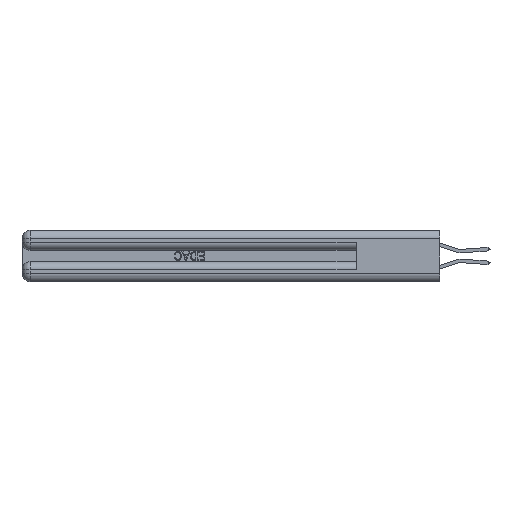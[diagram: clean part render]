
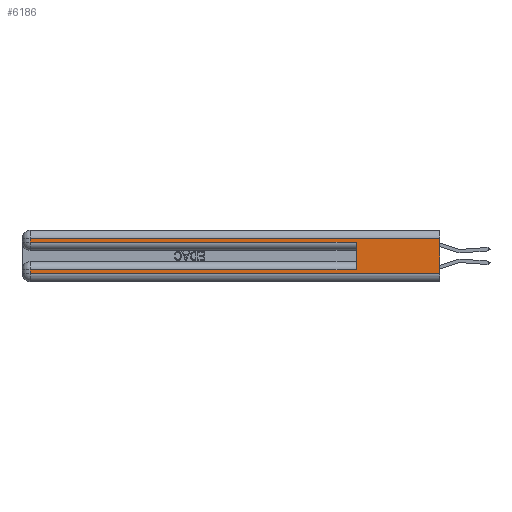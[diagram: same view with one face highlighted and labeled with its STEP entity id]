
A CAD part, left-side view. The second image highlights one B-rep face of the part: STEP entity #6186.
In plain terms, the highlighted planar face has unit normal (-1, 0, 0).
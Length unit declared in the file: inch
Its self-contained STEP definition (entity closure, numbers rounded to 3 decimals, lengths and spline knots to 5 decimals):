
#1685 = VERTEX_POINT ( 'NONE', #13729 ) ;
#1734 = ORIENTED_EDGE ( 'NONE', *, *, #13309, .T. ) ;
#2206 = DIRECTION ( 'NONE',  ( 0., 1., 0. ) ) ;
#2446 = DIRECTION ( 'NONE',  ( 1., 0., 0. ) ) ;
#2831 = EDGE_CURVE ( 'NONE', #9744, #1685, #5831, .T. ) ;
#3284 = VECTOR ( 'NONE', #41558, 39.37008 ) ;
#4957 = CARTESIAN_POINT ( 'NONE',  ( 0., 0.6, 0.085 ) ) ;
#5831 = LINE ( 'NONE', #7526, #36513 ) ;
#6186 = ADVANCED_FACE ( 'NONE', ( #16926 ), #17449, .F. ) ;
#6455 = VECTOR ( 'NONE', #2206, 39.37008 ) ;
#7526 = CARTESIAN_POINT ( 'NONE',  ( 0., 0., 0.285 ) ) ;
#8013 = LINE ( 'NONE', #31637, #43025 ) ;
#9462 = EDGE_CURVE ( 'NONE', #42711, #1685, #14419, .T. ) ;
#9478 = DIRECTION ( 'NONE',  ( 0., 0., -1. ) ) ;
#9744 = VERTEX_POINT ( 'NONE', #45219 ) ;
#9924 = DIRECTION ( 'NONE',  ( 0., 0., -1. ) ) ;
#10524 = ORIENTED_EDGE ( 'NONE', *, *, #30160, .T. ) ;
#10572 = LINE ( 'NONE', #27917, #3284 ) ;
#11528 = CARTESIAN_POINT ( 'NONE',  ( 0., 2.94, 0.31 ) ) ;
#11798 = DIRECTION ( 'NONE',  ( 0., 0., -1. ) ) ;
#12547 = CARTESIAN_POINT ( 'NONE',  ( 0., 0., 0.31 ) ) ;
#13142 = ORIENTED_EDGE ( 'NONE', *, *, #29932, .F. ) ;
#13309 = EDGE_CURVE ( 'NONE', #18652, #15798, #10572, .T. ) ;
#13339 = ORIENTED_EDGE ( 'NONE', *, *, #23525, .T. ) ;
#13513 = AXIS2_PLACEMENT_3D ( 'NONE', #31242, #2446, #9924 ) ;
#13729 = CARTESIAN_POINT ( 'NONE',  ( 0., 0.6, 0.285 ) ) ;
#14407 = LINE ( 'NONE', #34287, #41132 ) ;
#14419 = LINE ( 'NONE', #24568, #29417 ) ;
#15032 = EDGE_LOOP ( 'NONE', ( #13142, #20620, #34913, #41069, #33979, #13339, #10524, #1734 ) ) ;
#15798 = VERTEX_POINT ( 'NONE', #44072 ) ;
#16926 = FACE_OUTER_BOUND ( 'NONE', #15032, .T. ) ;
#17034 = VERTEX_POINT ( 'NONE', #35215 ) ;
#17332 = EDGE_CURVE ( 'NONE', #25956, #36977, #25423, .T. ) ;
#17449 = PLANE ( 'NONE',  #13513 ) ;
#17613 = VECTOR ( 'NONE', #9478, 39.37008 ) ;
#17676 = EDGE_CURVE ( 'NONE', #36977, #9744, #28126, .T. ) ;
#18652 = VERTEX_POINT ( 'NONE', #27134 ) ;
#20620 = ORIENTED_EDGE ( 'NONE', *, *, #17332, .T. ) ;
#22698 = VECTOR ( 'NONE', #11798, 39.37008 ) ;
#23525 = EDGE_CURVE ( 'NONE', #42711, #17034, #8013, .T. ) ;
#24320 = DIRECTION ( 'NONE',  ( 0., 1., 0. ) ) ;
#24398 = CARTESIAN_POINT ( 'NONE',  ( 0., 0., 0.31 ) ) ;
#24568 = CARTESIAN_POINT ( 'NONE',  ( 0., 0.6, 0.145 ) ) ;
#25423 = LINE ( 'NONE', #12547, #6455 ) ;
#25956 = VERTEX_POINT ( 'NONE', #24398 ) ;
#26805 = DIRECTION ( 'NONE',  ( 0., 0., -1. ) ) ;
#26938 = CARTESIAN_POINT ( 'NONE',  ( 0., 2.94, 0.37 ) ) ;
#27134 = CARTESIAN_POINT ( 'NONE',  ( 0., 2.94, 0.06 ) ) ;
#27917 = CARTESIAN_POINT ( 'NONE',  ( 0., 0., 0.06 ) ) ;
#28126 = LINE ( 'NONE', #26938, #17613 ) ;
#28218 = DIRECTION ( 'NONE',  ( 0., -1., 0. ) ) ;
#29417 = VECTOR ( 'NONE', #45500, 39.37008 ) ;
#29932 = EDGE_CURVE ( 'NONE', #25956, #15798, #14407, .T. ) ;
#30160 = EDGE_CURVE ( 'NONE', #17034, #18652, #44375, .T. ) ;
#31242 = CARTESIAN_POINT ( 'NONE',  ( 0., 0., 0.37 ) ) ;
#31637 = CARTESIAN_POINT ( 'NONE',  ( 0., 0., 0.085 ) ) ;
#33979 = ORIENTED_EDGE ( 'NONE', *, *, #9462, .F. ) ;
#34287 = CARTESIAN_POINT ( 'NONE',  ( 0., 0., 0.37 ) ) ;
#34913 = ORIENTED_EDGE ( 'NONE', *, *, #17676, .T. ) ;
#35215 = CARTESIAN_POINT ( 'NONE',  ( 0., 2.94, 0.085 ) ) ;
#36513 = VECTOR ( 'NONE', #28218, 39.37008 ) ;
#36688 = CARTESIAN_POINT ( 'NONE',  ( 0., 2.94, 0.37 ) ) ;
#36977 = VERTEX_POINT ( 'NONE', #11528 ) ;
#41069 = ORIENTED_EDGE ( 'NONE', *, *, #2831, .T. ) ;
#41132 = VECTOR ( 'NONE', #26805, 39.37008 ) ;
#41558 = DIRECTION ( 'NONE',  ( 0., -1., 0. ) ) ;
#42711 = VERTEX_POINT ( 'NONE', #4957 ) ;
#43025 = VECTOR ( 'NONE', #24320, 39.37008 ) ;
#44072 = CARTESIAN_POINT ( 'NONE',  ( 0., 0., 0.06 ) ) ;
#44375 = LINE ( 'NONE', #36688, #22698 ) ;
#45219 = CARTESIAN_POINT ( 'NONE',  ( 0., 2.94, 0.285 ) ) ;
#45500 = DIRECTION ( 'NONE',  ( 0., 0., 1. ) ) ;
